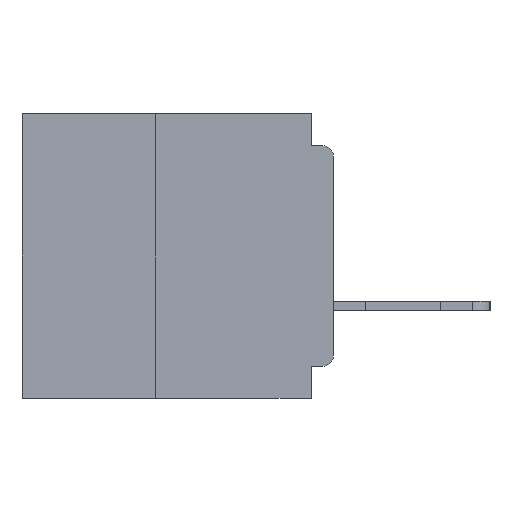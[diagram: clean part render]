
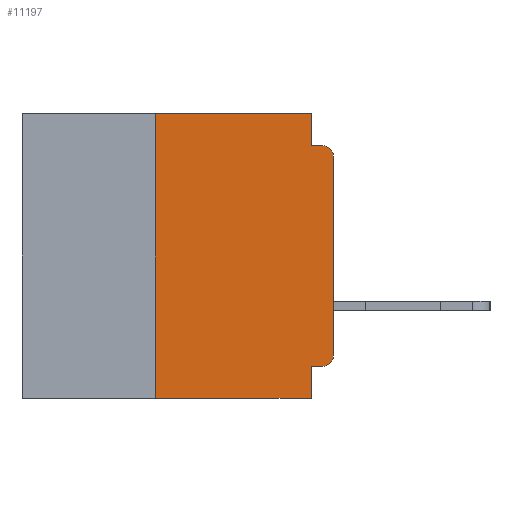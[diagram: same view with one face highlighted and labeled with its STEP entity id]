
A CAD part, left-side view. The second image highlights one B-rep face of the part: STEP entity #11197.
In plain terms, the highlighted planar face has unit normal (-1, 0, 0).
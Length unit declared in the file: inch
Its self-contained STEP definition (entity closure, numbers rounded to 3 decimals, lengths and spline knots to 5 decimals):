
#98 = LINE ( 'NONE', #32942, #46159 ) ;
#635 = EDGE_CURVE ( 'NONE', #50466, #17611, #38982, .T. ) ;
#1447 = LINE ( 'NONE', #28329, #23720 ) ;
#1659 = DIRECTION ( 'NONE',  ( 0., 0., -1. ) ) ;
#1891 = VECTOR ( 'NONE', #29450, 39.37008 ) ;
#1916 = CARTESIAN_POINT ( 'NONE',  ( 0., 0.015, -0.355 ) ) ;
#3046 = ORIENTED_EDGE ( 'NONE', *, *, #56113, .F. ) ;
#3160 = CARTESIAN_POINT ( 'NONE',  ( 0., 0.437, -0.4 ) ) ;
#3599 = VERTEX_POINT ( 'NONE', #11199 ) ;
#3616 = ORIENTED_EDGE ( 'NONE', *, *, #18217, .F. ) ;
#3739 = CARTESIAN_POINT ( 'NONE',  ( 0., 0., -0.355 ) ) ;
#5188 = ORIENTED_EDGE ( 'NONE', *, *, #7738, .T. ) ;
#5296 = DIRECTION ( 'NONE',  ( 0., 0., -1. ) ) ;
#5634 = CARTESIAN_POINT ( 'NONE',  ( 0., 0.031, -0.355 ) ) ;
#5942 = CIRCLE ( 'NONE', #31436, 0.015 ) ;
#6326 = DIRECTION ( 'NONE',  ( 0., 0., -1. ) ) ;
#6342 = DIRECTION ( 'NONE',  ( 0., 0., 1. ) ) ;
#7311 = DIRECTION ( 'NONE',  ( 0., 0., 1. ) ) ;
#7738 = EDGE_CURVE ( 'NONE', #17611, #26574, #8853, .T. ) ;
#8190 = DIRECTION ( 'NONE',  ( 0., 1., 0. ) ) ;
#8853 = LINE ( 'NONE', #32963, #44458 ) ;
#9552 = LINE ( 'NONE', #56224, #1891 ) ;
#10165 = ORIENTED_EDGE ( 'NONE', *, *, #39557, .F. ) ;
#11197 = ADVANCED_FACE ( 'NONE', ( #55884 ), #27467, .F. ) ;
#11199 = CARTESIAN_POINT ( 'NONE',  ( 0., 0.031, -0.4 ) ) ;
#14481 = CARTESIAN_POINT ( 'NONE',  ( 0., 0.015, -0.045 ) ) ;
#15061 = CARTESIAN_POINT ( 'NONE',  ( 0., 0.031, 0. ) ) ;
#16127 = ORIENTED_EDGE ( 'NONE', *, *, #26337, .F. ) ;
#16866 = VERTEX_POINT ( 'NONE', #14481 ) ;
#17310 = VERTEX_POINT ( 'NONE', #21821 ) ;
#17367 = DIRECTION ( 'NONE',  ( -1., 0., 0. ) ) ;
#17611 = VERTEX_POINT ( 'NONE', #19664 ) ;
#18217 = EDGE_CURVE ( 'NONE', #17310, #49217, #39353, .T. ) ;
#18903 = EDGE_CURVE ( 'NONE', #17310, #3599, #51129, .T. ) ;
#19212 = VECTOR ( 'NONE', #8190, 39.37008 ) ;
#19664 = CARTESIAN_POINT ( 'NONE',  ( 0., 0., -0.34 ) ) ;
#20599 = LINE ( 'NONE', #3739, #19212 ) ;
#21777 = VERTEX_POINT ( 'NONE', #45373 ) ;
#21821 = CARTESIAN_POINT ( 'NONE',  ( 0., 0.25, -0.4 ) ) ;
#23680 = VERTEX_POINT ( 'NONE', #15061 ) ;
#23720 = VECTOR ( 'NONE', #1659, 39.37008 ) ;
#25844 = AXIS2_PLACEMENT_3D ( 'NONE', #54078, #31936, #5296 ) ;
#26337 = EDGE_CURVE ( 'NONE', #21777, #16866, #57697, .T. ) ;
#26574 = VERTEX_POINT ( 'NONE', #55194 ) ;
#27467 = PLANE ( 'NONE',  #25844 ) ;
#28046 = EDGE_LOOP ( 'NONE', ( #5188, #50916, #16127, #52599, #45729, #3616, #56088, #3046, #10165, #45909 ) ) ;
#28329 = CARTESIAN_POINT ( 'NONE',  ( 0., 0.031, 0. ) ) ;
#29450 = DIRECTION ( 'NONE',  ( 0., -1., 0. ) ) ;
#29650 = EDGE_CURVE ( 'NONE', #23680, #21777, #1447, .T. ) ;
#30246 = VECTOR ( 'NONE', #7311, 39.37008 ) ;
#30380 = CARTESIAN_POINT ( 'NONE',  ( 0., 0.015, -0.34 ) ) ;
#30729 = VERTEX_POINT ( 'NONE', #5634 ) ;
#31319 = DIRECTION ( 'NONE',  ( 0., -1., 0. ) ) ;
#31436 = AXIS2_PLACEMENT_3D ( 'NONE', #44111, #17367, #48637 ) ;
#31936 = DIRECTION ( 'NONE',  ( 1., 0., 0. ) ) ;
#32050 = AXIS2_PLACEMENT_3D ( 'NONE', #30380, #57155, #36490 ) ;
#32942 = CARTESIAN_POINT ( 'NONE',  ( 0., 0.031, -0.4 ) ) ;
#32963 = CARTESIAN_POINT ( 'NONE',  ( 0., 0., 0. ) ) ;
#33962 = CARTESIAN_POINT ( 'NONE',  ( 0., 0.25, -0.4 ) ) ;
#34200 = EDGE_CURVE ( 'NONE', #49217, #23680, #9552, .T. ) ;
#36338 = CARTESIAN_POINT ( 'NONE',  ( 0., 0.25, 0. ) ) ;
#36490 = DIRECTION ( 'NONE',  ( 0., 0., -1. ) ) ;
#38982 = CIRCLE ( 'NONE', #32050, 0.015 ) ;
#39224 = VECTOR ( 'NONE', #52119, 39.37008 ) ;
#39353 = LINE ( 'NONE', #33962, #30246 ) ;
#39557 = EDGE_CURVE ( 'NONE', #50466, #30729, #20599, .T. ) ;
#39582 = EDGE_CURVE ( 'NONE', #26574, #16866, #5942, .T. ) ;
#44111 = CARTESIAN_POINT ( 'NONE',  ( 0., 0.015, -0.06 ) ) ;
#44458 = VECTOR ( 'NONE', #6342, 39.37008 ) ;
#44664 = CARTESIAN_POINT ( 'NONE',  ( 0., 0., -0.045 ) ) ;
#45373 = CARTESIAN_POINT ( 'NONE',  ( 0., 0.031, -0.045 ) ) ;
#45729 = ORIENTED_EDGE ( 'NONE', *, *, #34200, .F. ) ;
#45832 = VECTOR ( 'NONE', #31319, 39.37008 ) ;
#45909 = ORIENTED_EDGE ( 'NONE', *, *, #635, .T. ) ;
#46159 = VECTOR ( 'NONE', #6326, 39.37008 ) ;
#48637 = DIRECTION ( 'NONE',  ( 0., 0., -1. ) ) ;
#49217 = VERTEX_POINT ( 'NONE', #36338 ) ;
#50466 = VERTEX_POINT ( 'NONE', #1916 ) ;
#50916 = ORIENTED_EDGE ( 'NONE', *, *, #39582, .T. ) ;
#51129 = LINE ( 'NONE', #3160, #39224 ) ;
#52119 = DIRECTION ( 'NONE',  ( 0., -1., 0. ) ) ;
#52599 = ORIENTED_EDGE ( 'NONE', *, *, #29650, .F. ) ;
#54078 = CARTESIAN_POINT ( 'NONE',  ( 0., 0.437, 0. ) ) ;
#55194 = CARTESIAN_POINT ( 'NONE',  ( 0., 0., -0.06 ) ) ;
#55884 = FACE_OUTER_BOUND ( 'NONE', #28046, .T. ) ;
#56088 = ORIENTED_EDGE ( 'NONE', *, *, #18903, .T. ) ;
#56113 = EDGE_CURVE ( 'NONE', #30729, #3599, #98, .T. ) ;
#56224 = CARTESIAN_POINT ( 'NONE',  ( 0., 0.437, 0. ) ) ;
#57155 = DIRECTION ( 'NONE',  ( -1., 0., 0. ) ) ;
#57697 = LINE ( 'NONE', #44664, #45832 ) ;
